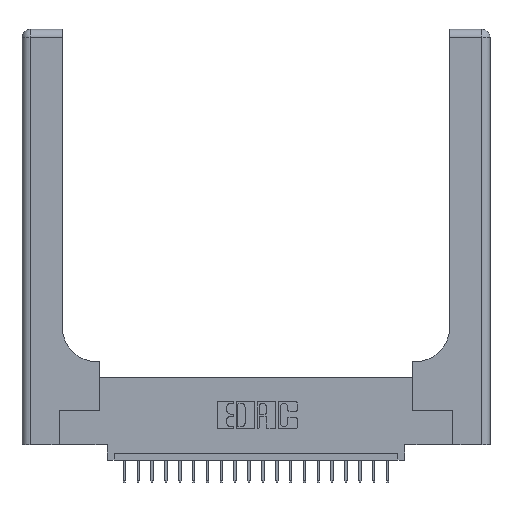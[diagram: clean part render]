
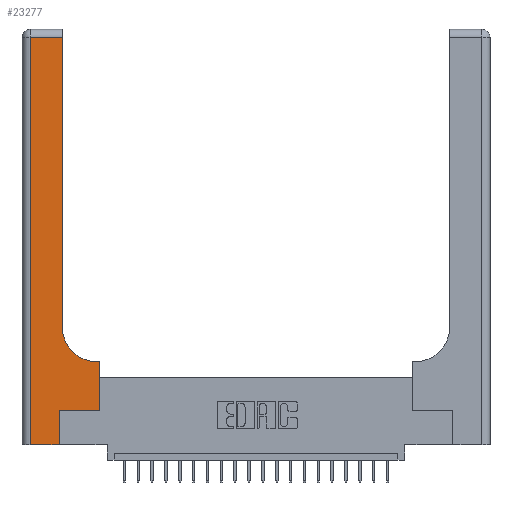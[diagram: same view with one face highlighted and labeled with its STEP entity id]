
A CAD part, top view. The second image highlights one B-rep face of the part: STEP entity #23277.
In plain terms, the highlighted planar face has unit normal (0, 0, 1).
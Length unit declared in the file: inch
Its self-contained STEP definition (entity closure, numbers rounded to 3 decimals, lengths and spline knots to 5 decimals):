
#288 = LINE ( 'NONE', #9504, #7731 ) ;
#969 = EDGE_CURVE ( 'NONE', #10103, #4252, #288, .T. ) ;
#1042 = PLANE ( 'NONE',  #9669 ) ;
#1407 = EDGE_CURVE ( 'NONE', #9811, #10398, #18667, .T. ) ;
#1686 = DIRECTION ( 'NONE',  ( 0., 1., 0. ) ) ;
#2525 = VERTEX_POINT ( 'NONE', #13876 ) ;
#2760 = VECTOR ( 'NONE', #12842, 39.37008 ) ;
#2851 = DIRECTION ( 'NONE',  ( 0., 1., 0. ) ) ;
#2859 = ORIENTED_EDGE ( 'NONE', *, *, #1407, .T. ) ;
#3465 = EDGE_CURVE ( 'NONE', #2525, #17929, #5934, .T. ) ;
#3538 = AXIS2_PLACEMENT_3D ( 'NONE', #5173, #14804, #11132 ) ;
#3583 = DIRECTION ( 'NONE',  ( -1., 0., 0. ) ) ;
#3606 = ORIENTED_EDGE ( 'NONE', *, *, #17737, .T. ) ;
#3683 = ORIENTED_EDGE ( 'NONE', *, *, #3465, .T. ) ;
#3795 = FACE_OUTER_BOUND ( 'NONE', #10795, .T. ) ;
#4252 = VERTEX_POINT ( 'NONE', #4289 ) ;
#4289 = CARTESIAN_POINT ( 'NONE',  ( 0.5415, 0.6, 0.37 ) ) ;
#4660 = VERTEX_POINT ( 'NONE', #18690 ) ;
#5060 = CARTESIAN_POINT ( 'NONE',  ( 0.269, 0.25, 0.37 ) ) ;
#5173 = CARTESIAN_POINT ( 'NONE',  ( 0.5415, 0.85, 0.37 ) ) ;
#5711 = VECTOR ( 'NONE', #7016, 39.37008 ) ;
#5771 = VECTOR ( 'NONE', #17407, 39.37008 ) ;
#5934 = LINE ( 'NONE', #19821, #2760 ) ;
#6119 = CARTESIAN_POINT ( 'NONE',  ( 0.2915, 2.94, 0.37 ) ) ;
#7016 = DIRECTION ( 'NONE',  ( 1., 0., 0. ) ) ;
#7731 = VECTOR ( 'NONE', #13239, 39.37008 ) ;
#7994 = CARTESIAN_POINT ( 'NONE',  ( 0.2915, 3., 0.37 ) ) ;
#8448 = CIRCLE ( 'NONE', #3538, 0.25 ) ;
#8635 = VERTEX_POINT ( 'NONE', #6119 ) ;
#8970 = CARTESIAN_POINT ( 'NONE',  ( 0.269, 0., 0.37 ) ) ;
#9360 = CARTESIAN_POINT ( 'NONE',  ( 0.5585, 0.25, 0.37 ) ) ;
#9453 = EDGE_CURVE ( 'NONE', #4660, #9811, #23081, .T. ) ;
#9504 = CARTESIAN_POINT ( 'NONE',  ( 0.2915, 0.6, 0.37 ) ) ;
#9669 = AXIS2_PLACEMENT_3D ( 'NONE', #19209, #10443, #19452 ) ;
#9706 = VECTOR ( 'NONE', #2851, 39.37008 ) ;
#9811 = VERTEX_POINT ( 'NONE', #19647 ) ;
#9928 = DIRECTION ( 'NONE',  ( 0., 1., 0. ) ) ;
#10103 = VERTEX_POINT ( 'NONE', #12012 ) ;
#10398 = VERTEX_POINT ( 'NONE', #9360 ) ;
#10443 = DIRECTION ( 'NONE',  ( 0., 0., -1. ) ) ;
#10480 = LINE ( 'NONE', #17038, #21698 ) ;
#10795 = EDGE_LOOP ( 'NONE', ( #14078, #19304, #3683, #3606, #16951, #2859, #13136, #14937, #12075 ) ) ;
#11132 = DIRECTION ( 'NONE',  ( 1., 0., 0. ) ) ;
#11943 = LINE ( 'NONE', #7994, #9706 ) ;
#12012 = CARTESIAN_POINT ( 'NONE',  ( 0.5585, 0.6, 0.37 ) ) ;
#12075 = ORIENTED_EDGE ( 'NONE', *, *, #14301, .T. ) ;
#12842 = DIRECTION ( 'NONE',  ( 0., -1., 0. ) ) ;
#12936 = VECTOR ( 'NONE', #3583, 39.37008 ) ;
#13050 = CARTESIAN_POINT ( 'NONE',  ( 0.06, 0., 0.37 ) ) ;
#13136 = ORIENTED_EDGE ( 'NONE', *, *, #20767, .T. ) ;
#13239 = DIRECTION ( 'NONE',  ( -1., 0., 0. ) ) ;
#13876 = CARTESIAN_POINT ( 'NONE',  ( 0.06, 2.94, 0.37 ) ) ;
#14078 = ORIENTED_EDGE ( 'NONE', *, *, #18451, .T. ) ;
#14288 = EDGE_CURVE ( 'NONE', #8635, #2525, #14900, .T. ) ;
#14301 = EDGE_CURVE ( 'NONE', #4252, #20759, #8448, .T. ) ;
#14804 = DIRECTION ( 'NONE',  ( 0., 0., -1. ) ) ;
#14900 = LINE ( 'NONE', #21237, #12936 ) ;
#14937 = ORIENTED_EDGE ( 'NONE', *, *, #969, .T. ) ;
#15331 = LINE ( 'NONE', #20713, #5771 ) ;
#16951 = ORIENTED_EDGE ( 'NONE', *, *, #9453, .T. ) ;
#17038 = CARTESIAN_POINT ( 'NONE',  ( 0.5585, 0.25, 0.37 ) ) ;
#17407 = DIRECTION ( 'NONE',  ( 1., 0., 0. ) ) ;
#17737 = EDGE_CURVE ( 'NONE', #17929, #4660, #15331, .T. ) ;
#17929 = VERTEX_POINT ( 'NONE', #13050 ) ;
#18451 = EDGE_CURVE ( 'NONE', #20759, #8635, #11943, .T. ) ;
#18667 = LINE ( 'NONE', #5060, #5711 ) ;
#18690 = CARTESIAN_POINT ( 'NONE',  ( 0.269, 0., 0.37 ) ) ;
#19209 = CARTESIAN_POINT ( 'NONE',  ( 0., 3., 0.37 ) ) ;
#19304 = ORIENTED_EDGE ( 'NONE', *, *, #14288, .T. ) ;
#19452 = DIRECTION ( 'NONE',  ( -1., 0., 0. ) ) ;
#19647 = CARTESIAN_POINT ( 'NONE',  ( 0.269, 0.25, 0.37 ) ) ;
#19821 = CARTESIAN_POINT ( 'NONE',  ( 0.06, 3., 0.37 ) ) ;
#20358 = CARTESIAN_POINT ( 'NONE',  ( 0.2915, 0.85, 0.37 ) ) ;
#20713 = CARTESIAN_POINT ( 'NONE',  ( 0., 0., 0.37 ) ) ;
#20759 = VERTEX_POINT ( 'NONE', #20358 ) ;
#20767 = EDGE_CURVE ( 'NONE', #10398, #10103, #10480, .T. ) ;
#21237 = CARTESIAN_POINT ( 'NONE',  ( 0., 2.94, 0.37 ) ) ;
#21698 = VECTOR ( 'NONE', #9928, 39.37008 ) ;
#22811 = VECTOR ( 'NONE', #1686, 39.37008 ) ;
#23081 = LINE ( 'NONE', #8970, #22811 ) ;
#23277 = ADVANCED_FACE ( 'NONE', ( #3795 ), #1042, .F. ) ;
